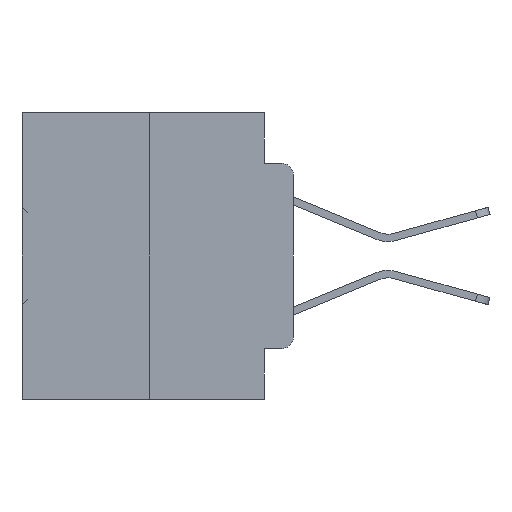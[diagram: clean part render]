
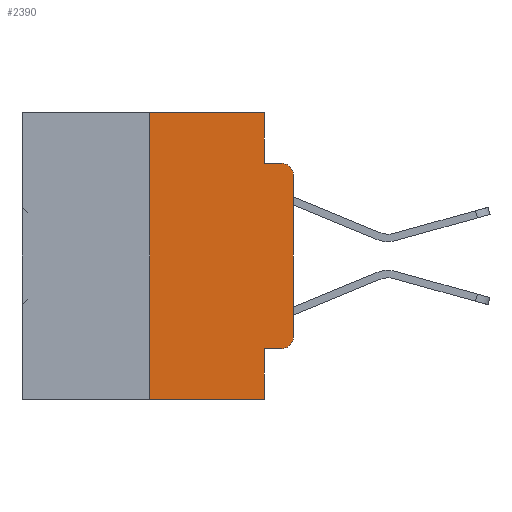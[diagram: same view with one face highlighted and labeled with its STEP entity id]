
A CAD part, left-side view. The second image highlights one B-rep face of the part: STEP entity #2390.
In plain terms, the highlighted planar face has unit normal (-1, 0, 0).
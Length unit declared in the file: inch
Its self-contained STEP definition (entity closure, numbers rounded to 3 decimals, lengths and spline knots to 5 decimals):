
#57 = ORIENTED_EDGE ( 'NONE', *, *, #2274, .T. ) ;
#396 = CIRCLE ( 'NONE', #17060, 0.02 ) ;
#832 = CARTESIAN_POINT ( 'NONE',  ( 0., 0.473, 0. ) ) ;
#1429 = LINE ( 'NONE', #11177, #31954 ) ;
#1439 = VERTEX_POINT ( 'NONE', #20595 ) ;
#1858 = DIRECTION ( 'NONE',  ( 1., 0., 0. ) ) ;
#2274 = EDGE_CURVE ( 'NONE', #26730, #21877, #33993, .T. ) ;
#2390 = ADVANCED_FACE ( 'NONE', ( #5799 ), #8423, .F. ) ;
#2420 = CARTESIAN_POINT ( 'NONE',  ( 0., 0.051, 0. ) ) ;
#2533 = DIRECTION ( 'NONE',  ( 0., -1., 0. ) ) ;
#3710 = LINE ( 'NONE', #2420, #10644 ) ;
#5105 = CARTESIAN_POINT ( 'NONE',  ( 0., 0.473, 0. ) ) ;
#5799 = FACE_OUTER_BOUND ( 'NONE', #29064, .T. ) ;
#6628 = ORIENTED_EDGE ( 'NONE', *, *, #37088, .T. ) ;
#6845 = DIRECTION ( 'NONE',  ( -1., 0., 0. ) ) ;
#8423 = PLANE ( 'NONE',  #19337 ) ;
#8444 = CARTESIAN_POINT ( 'NONE',  ( 0., 0.25, 0. ) ) ;
#9839 = ORIENTED_EDGE ( 'NONE', *, *, #34674, .T. ) ;
#10153 = VERTEX_POINT ( 'NONE', #12048 ) ;
#10644 = VECTOR ( 'NONE', #20201, 39.37008 ) ;
#10901 = EDGE_CURVE ( 'NONE', #23691, #26730, #396, .T. ) ;
#11177 = CARTESIAN_POINT ( 'NONE',  ( 0., 0.051, -0.0885 ) ) ;
#11633 = DIRECTION ( 'NONE',  ( 0., 0., -1. ) ) ;
#12048 = CARTESIAN_POINT ( 'NONE',  ( 0., 0.051, -0.5 ) ) ;
#12625 = ORIENTED_EDGE ( 'NONE', *, *, #24861, .F. ) ;
#13041 = CARTESIAN_POINT ( 'NONE',  ( 0., 0.02, -0.3915 ) ) ;
#14111 = DIRECTION ( 'NONE',  ( 0., 0., 1. ) ) ;
#15213 = EDGE_CURVE ( 'NONE', #28126, #29121, #26353, .T. ) ;
#15891 = CARTESIAN_POINT ( 'NONE',  ( 0., 0.051, 0. ) ) ;
#16072 = DIRECTION ( 'NONE',  ( 0., 0., -1. ) ) ;
#16120 = CARTESIAN_POINT ( 'NONE',  ( 0., 0.25, -0.5 ) ) ;
#16489 = DIRECTION ( 'NONE',  ( 0., -1., 0. ) ) ;
#17060 = AXIS2_PLACEMENT_3D ( 'NONE', #13041, #33701, #16072 ) ;
#17337 = ORIENTED_EDGE ( 'NONE', *, *, #22895, .F. ) ;
#17500 = DIRECTION ( 'NONE',  ( 0., -1., 0. ) ) ;
#17588 = VECTOR ( 'NONE', #34539, 39.37008 ) ;
#17778 = ORIENTED_EDGE ( 'NONE', *, *, #32695, .F. ) ;
#19337 = AXIS2_PLACEMENT_3D ( 'NONE', #832, #1858, #36748 ) ;
#19648 = ORIENTED_EDGE ( 'NONE', *, *, #30737, .F. ) ;
#20201 = DIRECTION ( 'NONE',  ( 0., 0., -1. ) ) ;
#20595 = CARTESIAN_POINT ( 'NONE',  ( 0., 0.02, -0.0885 ) ) ;
#20911 = EDGE_CURVE ( 'NONE', #30118, #23691, #31800, .T. ) ;
#21083 = VECTOR ( 'NONE', #11633, 39.37008 ) ;
#21473 = CARTESIAN_POINT ( 'NONE',  ( 0., 0.02, -0.4115 ) ) ;
#21501 = VECTOR ( 'NONE', #16489, 39.37008 ) ;
#21877 = VERTEX_POINT ( 'NONE', #24552 ) ;
#22166 = CIRCLE ( 'NONE', #33643, 0.02 ) ;
#22895 = EDGE_CURVE ( 'NONE', #30118, #10153, #37557, .T. ) ;
#23290 = VERTEX_POINT ( 'NONE', #36968 ) ;
#23691 = VERTEX_POINT ( 'NONE', #21473 ) ;
#23990 = VECTOR ( 'NONE', #17500, 39.37008 ) ;
#24096 = CARTESIAN_POINT ( 'NONE',  ( 0., 0.051, -0.4115 ) ) ;
#24552 = CARTESIAN_POINT ( 'NONE',  ( 0., 0., -0.1085 ) ) ;
#24594 = CARTESIAN_POINT ( 'NONE',  ( 0., 0.02, -0.1085 ) ) ;
#24798 = CARTESIAN_POINT ( 'NONE',  ( 0., 0., 0. ) ) ;
#24861 = EDGE_CURVE ( 'NONE', #36490, #28126, #26434, .T. ) ;
#25186 = ORIENTED_EDGE ( 'NONE', *, *, #10901, .T. ) ;
#25287 = VECTOR ( 'NONE', #34217, 39.37008 ) ;
#26353 = LINE ( 'NONE', #5105, #17588 ) ;
#26434 = LINE ( 'NONE', #31757, #27335 ) ;
#26730 = VERTEX_POINT ( 'NONE', #32149 ) ;
#27335 = VECTOR ( 'NONE', #14111, 39.37008 ) ;
#27530 = DIRECTION ( 'NONE',  ( 0., 0., -1. ) ) ;
#28126 = VERTEX_POINT ( 'NONE', #8444 ) ;
#29064 = EDGE_LOOP ( 'NONE', ( #57, #9839, #17778, #19648, #35242, #12625, #6628, #17337, #30204, #25186 ) ) ;
#29121 = VERTEX_POINT ( 'NONE', #15891 ) ;
#29366 = CARTESIAN_POINT ( 'NONE',  ( 0., 0.051, 0. ) ) ;
#30118 = VERTEX_POINT ( 'NONE', #24096 ) ;
#30204 = ORIENTED_EDGE ( 'NONE', *, *, #20911, .T. ) ;
#30737 = EDGE_CURVE ( 'NONE', #29121, #23290, #3710, .T. ) ;
#31757 = CARTESIAN_POINT ( 'NONE',  ( 0., 0.25, 0. ) ) ;
#31800 = LINE ( 'NONE', #37868, #23990 ) ;
#31954 = VECTOR ( 'NONE', #2533, 39.37008 ) ;
#32149 = CARTESIAN_POINT ( 'NONE',  ( 0., 0., -0.3915 ) ) ;
#32695 = EDGE_CURVE ( 'NONE', #23290, #1439, #1429, .T. ) ;
#33643 = AXIS2_PLACEMENT_3D ( 'NONE', #24594, #6845, #27530 ) ;
#33701 = DIRECTION ( 'NONE',  ( -1., 0., 0. ) ) ;
#33993 = LINE ( 'NONE', #24798, #25287 ) ;
#34087 = CARTESIAN_POINT ( 'NONE',  ( 0., 0.473, -0.5 ) ) ;
#34217 = DIRECTION ( 'NONE',  ( 0., 0., 1. ) ) ;
#34539 = DIRECTION ( 'NONE',  ( 0., -1., 0. ) ) ;
#34674 = EDGE_CURVE ( 'NONE', #21877, #1439, #22166, .T. ) ;
#35242 = ORIENTED_EDGE ( 'NONE', *, *, #15213, .F. ) ;
#36490 = VERTEX_POINT ( 'NONE', #16120 ) ;
#36748 = DIRECTION ( 'NONE',  ( 0., 0., -1. ) ) ;
#36968 = CARTESIAN_POINT ( 'NONE',  ( 0., 0.051, -0.0885 ) ) ;
#37053 = LINE ( 'NONE', #34087, #21501 ) ;
#37088 = EDGE_CURVE ( 'NONE', #36490, #10153, #37053, .T. ) ;
#37557 = LINE ( 'NONE', #29366, #21083 ) ;
#37868 = CARTESIAN_POINT ( 'NONE',  ( 0., 0.051, -0.4115 ) ) ;
